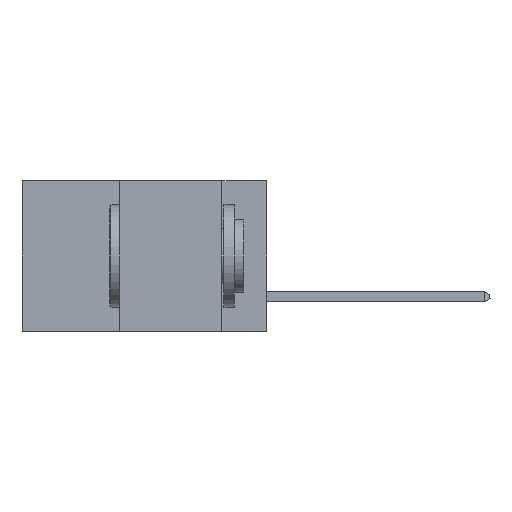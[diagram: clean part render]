
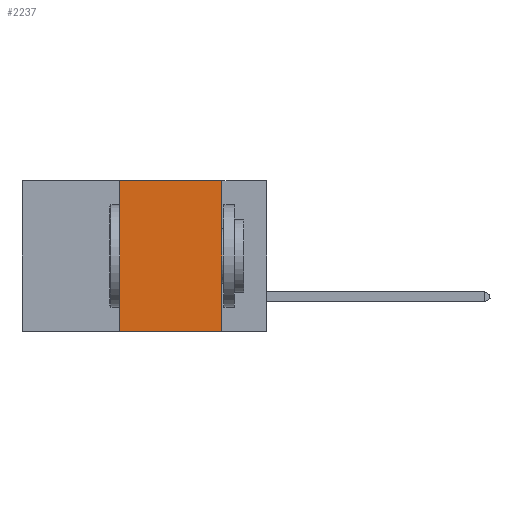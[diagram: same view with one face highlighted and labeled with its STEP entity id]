
A CAD part, left-side view. The second image highlights one B-rep face of the part: STEP entity #2237.
In plain terms, the highlighted planar face has unit normal (-1, 0, 0).
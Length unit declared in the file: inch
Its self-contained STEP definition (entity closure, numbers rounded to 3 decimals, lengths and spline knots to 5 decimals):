
#1166 = ORIENTED_EDGE ( 'NONE', *, *, #20527, .F. ) ;
#1181 = LINE ( 'NONE', #7809, #27377 ) ;
#2237 = ADVANCED_FACE ( 'NONE', ( #11114 ), #23761, .F. ) ;
#2891 = LINE ( 'NONE', #24176, #4372 ) ;
#3665 = DIRECTION ( 'NONE',  ( 0., -1., 0. ) ) ;
#4220 = ORIENTED_EDGE ( 'NONE', *, *, #22983, .T. ) ;
#4372 = VECTOR ( 'NONE', #24489, 39.37008 ) ;
#4808 = LINE ( 'NONE', #20265, #9256 ) ;
#5517 = ORIENTED_EDGE ( 'NONE', *, *, #12049, .F. ) ;
#5617 = EDGE_LOOP ( 'NONE', ( #1166, #27935, #5517, #4220 ) ) ;
#5987 = VERTEX_POINT ( 'NONE', #7544 ) ;
#7544 = CARTESIAN_POINT ( 'NONE',  ( 0., 0.11, -0.37 ) ) ;
#7809 = CARTESIAN_POINT ( 'NONE',  ( 0., 0.11, 0. ) ) ;
#7972 = AXIS2_PLACEMENT_3D ( 'NONE', #14244, #9574, #11975 ) ;
#8391 = EDGE_CURVE ( 'NONE', #10036, #22673, #4808, .T. ) ;
#9256 = VECTOR ( 'NONE', #3665, 39.37008 ) ;
#9574 = DIRECTION ( 'NONE',  ( 1., 0., 0. ) ) ;
#10036 = VERTEX_POINT ( 'NONE', #16969 ) ;
#10366 = VERTEX_POINT ( 'NONE', #14010 ) ;
#10418 = VECTOR ( 'NONE', #20288, 39.37008 ) ;
#11114 = FACE_OUTER_BOUND ( 'NONE', #5617, .T. ) ;
#11975 = DIRECTION ( 'NONE',  ( 0., 0., -1. ) ) ;
#12049 = EDGE_CURVE ( 'NONE', #10366, #10036, #24377, .T. ) ;
#14010 = CARTESIAN_POINT ( 'NONE',  ( 0., 0.36, -0.37 ) ) ;
#14244 = CARTESIAN_POINT ( 'NONE',  ( 0., 0.6, 0. ) ) ;
#15504 = CARTESIAN_POINT ( 'NONE',  ( 0., 0.11, 0. ) ) ;
#16969 = CARTESIAN_POINT ( 'NONE',  ( 0., 0.36, 0. ) ) ;
#20265 = CARTESIAN_POINT ( 'NONE',  ( 0., 0.6, 0. ) ) ;
#20288 = DIRECTION ( 'NONE',  ( 0., 0., 1. ) ) ;
#20527 = EDGE_CURVE ( 'NONE', #22673, #5987, #1181, .T. ) ;
#20675 = CARTESIAN_POINT ( 'NONE',  ( 0., 0.36, 0. ) ) ;
#22673 = VERTEX_POINT ( 'NONE', #15504 ) ;
#22983 = EDGE_CURVE ( 'NONE', #10366, #5987, #2891, .T. ) ;
#23761 = PLANE ( 'NONE',  #7972 ) ;
#24176 = CARTESIAN_POINT ( 'NONE',  ( 0., 0.6, -0.37 ) ) ;
#24377 = LINE ( 'NONE', #20675, #10418 ) ;
#24474 = DIRECTION ( 'NONE',  ( 0., 0., -1. ) ) ;
#24489 = DIRECTION ( 'NONE',  ( 0., -1., 0. ) ) ;
#27377 = VECTOR ( 'NONE', #24474, 39.37008 ) ;
#27935 = ORIENTED_EDGE ( 'NONE', *, *, #8391, .F. ) ;
